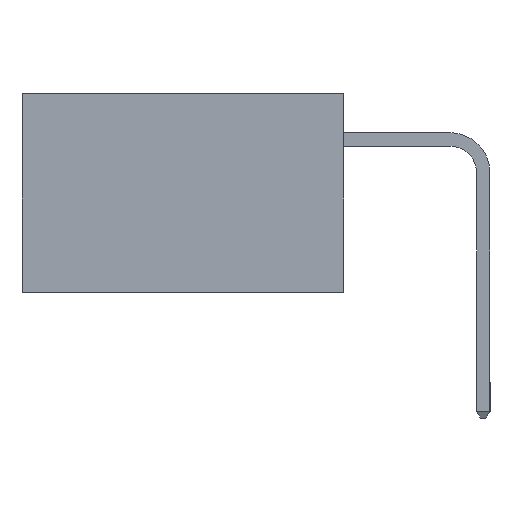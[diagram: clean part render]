
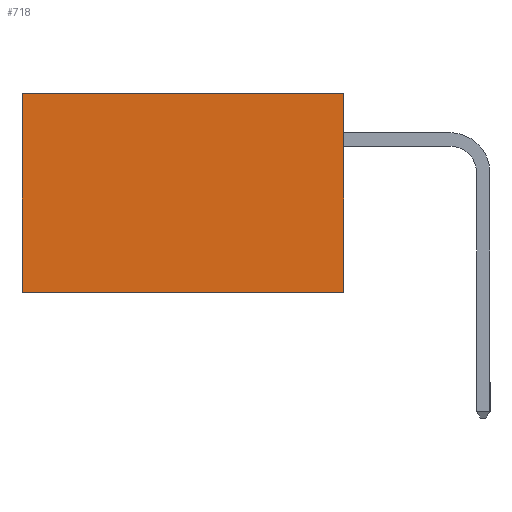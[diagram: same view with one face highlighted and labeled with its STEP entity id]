
A CAD part, left-side view. The second image highlights one B-rep face of the part: STEP entity #718.
In plain terms, the highlighted planar face has unit normal (-1, 0, 0).
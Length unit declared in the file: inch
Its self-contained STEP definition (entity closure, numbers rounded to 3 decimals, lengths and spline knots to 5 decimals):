
#523 = ORIENTED_EDGE ( 'NONE', *, *, #23810, .T. ) ;
#718 = ADVANCED_FACE ( 'NONE', ( #4374 ), #4874, .F. ) ;
#2147 = LINE ( 'NONE', #6461, #8245 ) ;
#4374 = FACE_OUTER_BOUND ( 'NONE', #16050, .T. ) ;
#4574 = VERTEX_POINT ( 'NONE', #18314 ) ;
#4874 = PLANE ( 'NONE',  #25784 ) ;
#5044 = DIRECTION ( 'NONE',  ( 0., 0., -1. ) ) ;
#6461 = CARTESIAN_POINT ( 'NONE',  ( 0.298, 0.6, 0. ) ) ;
#8245 = VECTOR ( 'NONE', #18798, 39.37008 ) ;
#9185 = LINE ( 'NONE', #23935, #10491 ) ;
#9502 = DIRECTION ( 'NONE',  ( 0., 1., 0. ) ) ;
#9741 = ORIENTED_EDGE ( 'NONE', *, *, #22865, .F. ) ;
#10491 = VECTOR ( 'NONE', #9502, 39.37008 ) ;
#10716 = VECTOR ( 'NONE', #23628, 39.37008 ) ;
#11202 = CARTESIAN_POINT ( 'NONE',  ( 0.298, 0., -0.37 ) ) ;
#12498 = LINE ( 'NONE', #18767, #22802 ) ;
#13393 = CARTESIAN_POINT ( 'NONE',  ( 0.298, 0., 0. ) ) ;
#14321 = VERTEX_POINT ( 'NONE', #23947 ) ;
#14652 = EDGE_CURVE ( 'NONE', #14321, #4574, #2147, .T. ) ;
#15435 = VERTEX_POINT ( 'NONE', #13393 ) ;
#15541 = ORIENTED_EDGE ( 'NONE', *, *, #14652, .T. ) ;
#16050 = EDGE_LOOP ( 'NONE', ( #15541, #26591, #9741, #523 ) ) ;
#16203 = LINE ( 'NONE', #21555, #10716 ) ;
#17166 = VERTEX_POINT ( 'NONE', #11202 ) ;
#18314 = CARTESIAN_POINT ( 'NONE',  ( 0.298, 0.6, -0.37 ) ) ;
#18517 = DIRECTION ( 'NONE',  ( 1., 0., 0. ) ) ;
#18551 = CARTESIAN_POINT ( 'NONE',  ( 0.298, 0., 0. ) ) ;
#18767 = CARTESIAN_POINT ( 'NONE',  ( 0.298, 0., 0. ) ) ;
#18798 = DIRECTION ( 'NONE',  ( 0., 0., -1. ) ) ;
#19907 = EDGE_CURVE ( 'NONE', #17166, #4574, #16203, .T. ) ;
#20838 = DIRECTION ( 'NONE',  ( 0., 0., -1. ) ) ;
#21555 = CARTESIAN_POINT ( 'NONE',  ( 0.298, 0., -0.37 ) ) ;
#22802 = VECTOR ( 'NONE', #20838, 39.37008 ) ;
#22865 = EDGE_CURVE ( 'NONE', #15435, #17166, #12498, .T. ) ;
#23628 = DIRECTION ( 'NONE',  ( 0., 1., 0. ) ) ;
#23810 = EDGE_CURVE ( 'NONE', #15435, #14321, #9185, .T. ) ;
#23935 = CARTESIAN_POINT ( 'NONE',  ( 0.298, 0., 0. ) ) ;
#23947 = CARTESIAN_POINT ( 'NONE',  ( 0.298, 0.6, 0. ) ) ;
#25784 = AXIS2_PLACEMENT_3D ( 'NONE', #18551, #18517, #5044 ) ;
#26591 = ORIENTED_EDGE ( 'NONE', *, *, #19907, .F. ) ;
